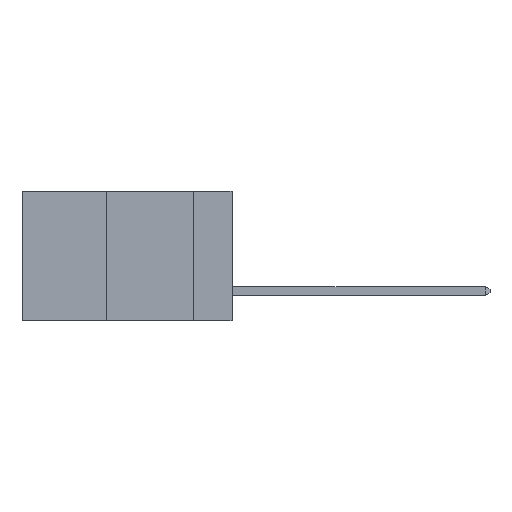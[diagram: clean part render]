
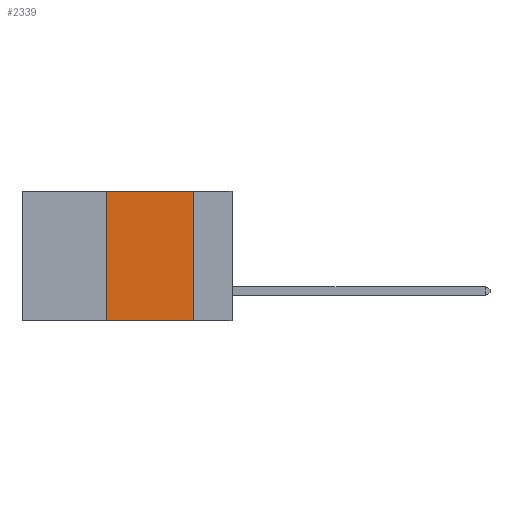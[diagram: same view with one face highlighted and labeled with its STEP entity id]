
A CAD part, left-side view. The second image highlights one B-rep face of the part: STEP entity #2339.
In plain terms, the highlighted planar face has unit normal (-1, 0, 0).
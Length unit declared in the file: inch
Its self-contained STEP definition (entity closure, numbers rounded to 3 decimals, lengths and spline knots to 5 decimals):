
#438 = FACE_OUTER_BOUND ( 'NONE', #2575, .T. ) ;
#559 = VECTOR ( 'NONE', #10859, 39.37008 ) ;
#2121 = LINE ( 'NONE', #10003, #6636 ) ;
#2339 = ADVANCED_FACE ( 'NONE', ( #438 ), #5344, .F. ) ;
#2460 = VECTOR ( 'NONE', #13101, 39.37008 ) ;
#2575 = EDGE_LOOP ( 'NONE', ( #18878, #14374, #21274, #12309 ) ) ;
#3544 = CARTESIAN_POINT ( 'NONE',  ( 0., 0.36, 0. ) ) ;
#3555 = CARTESIAN_POINT ( 'NONE',  ( 0., 0.36, 0. ) ) ;
#3656 = AXIS2_PLACEMENT_3D ( 'NONE', #20502, #9144, #22429 ) ;
#4883 = EDGE_CURVE ( 'NONE', #8825, #7179, #2121, .T. ) ;
#5110 = LINE ( 'NONE', #22276, #559 ) ;
#5344 = PLANE ( 'NONE',  #3656 ) ;
#6636 = VECTOR ( 'NONE', #8114, 39.37008 ) ;
#7056 = EDGE_CURVE ( 'NONE', #22369, #13555, #7557, .T. ) ;
#7179 = VERTEX_POINT ( 'NONE', #19219 ) ;
#7557 = LINE ( 'NONE', #20734, #2460 ) ;
#8114 = DIRECTION ( 'NONE',  ( 0., -1., 0. ) ) ;
#8746 = CARTESIAN_POINT ( 'NONE',  ( 0., 0.11, -0.37 ) ) ;
#8825 = VERTEX_POINT ( 'NONE', #3544 ) ;
#9144 = DIRECTION ( 'NONE',  ( 1., 0., 0. ) ) ;
#10003 = CARTESIAN_POINT ( 'NONE',  ( 0., 0.6, 0. ) ) ;
#10527 = LINE ( 'NONE', #3555, #23237 ) ;
#10859 = DIRECTION ( 'NONE',  ( 0., 0., -1. ) ) ;
#11160 = DIRECTION ( 'NONE',  ( 0., 0., 1. ) ) ;
#12077 = EDGE_CURVE ( 'NONE', #22369, #8825, #10527, .T. ) ;
#12309 = ORIENTED_EDGE ( 'NONE', *, *, #7056, .T. ) ;
#13101 = DIRECTION ( 'NONE',  ( 0., -1., 0. ) ) ;
#13555 = VERTEX_POINT ( 'NONE', #8746 ) ;
#14374 = ORIENTED_EDGE ( 'NONE', *, *, #4883, .F. ) ;
#16238 = CARTESIAN_POINT ( 'NONE',  ( 0., 0.36, -0.37 ) ) ;
#18878 = ORIENTED_EDGE ( 'NONE', *, *, #21042, .F. ) ;
#19219 = CARTESIAN_POINT ( 'NONE',  ( 0., 0.11, 0. ) ) ;
#20502 = CARTESIAN_POINT ( 'NONE',  ( 0., 0.6, 0. ) ) ;
#20734 = CARTESIAN_POINT ( 'NONE',  ( 0., 0.6, -0.37 ) ) ;
#21042 = EDGE_CURVE ( 'NONE', #7179, #13555, #5110, .T. ) ;
#21274 = ORIENTED_EDGE ( 'NONE', *, *, #12077, .F. ) ;
#22276 = CARTESIAN_POINT ( 'NONE',  ( 0., 0.11, 0. ) ) ;
#22369 = VERTEX_POINT ( 'NONE', #16238 ) ;
#22429 = DIRECTION ( 'NONE',  ( 0., 0., -1. ) ) ;
#23237 = VECTOR ( 'NONE', #11160, 39.37008 ) ;
